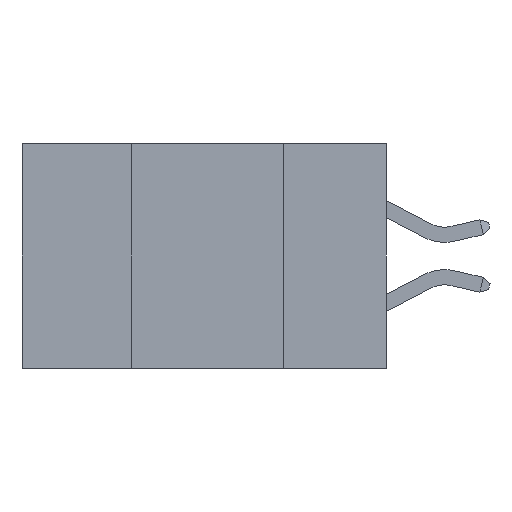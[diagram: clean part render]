
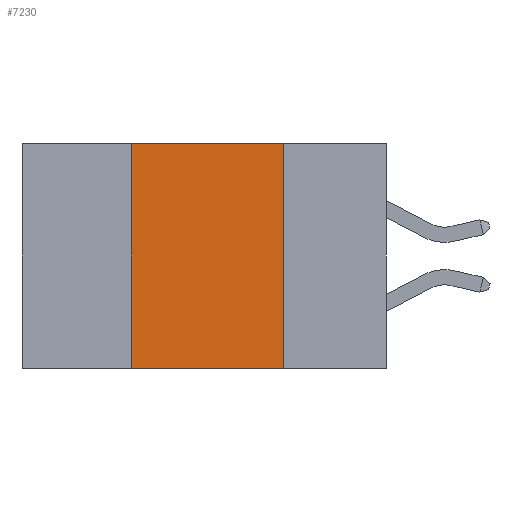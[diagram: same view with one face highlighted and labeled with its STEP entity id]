
A CAD part, left-side view. The second image highlights one B-rep face of the part: STEP entity #7230.
In plain terms, the highlighted planar face has unit normal (-1, 0, 0).
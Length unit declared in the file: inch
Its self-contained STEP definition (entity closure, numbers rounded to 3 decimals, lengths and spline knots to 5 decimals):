
#641 = EDGE_LOOP ( 'NONE', ( #16654, #2404, #4590, #13227 ) ) ;
#651 = EDGE_CURVE ( 'NONE', #1362, #14992, #16587, .T. ) ;
#781 = CARTESIAN_POINT ( 'NONE',  ( 0., 0.17, 0. ) ) ;
#1362 = VERTEX_POINT ( 'NONE', #781 ) ;
#2283 = DIRECTION ( 'NONE',  ( 0., -1., 0. ) ) ;
#2404 = ORIENTED_EDGE ( 'NONE', *, *, #9016, .F. ) ;
#4414 = DIRECTION ( 'NONE',  ( 0., 0., -1. ) ) ;
#4590 = ORIENTED_EDGE ( 'NONE', *, *, #5785, .F. ) ;
#5785 = EDGE_CURVE ( 'NONE', #12525, #13629, #13526, .T. ) ;
#5913 = CARTESIAN_POINT ( 'NONE',  ( 0., 0.42, -0.37 ) ) ;
#7230 = ADVANCED_FACE ( 'NONE', ( #9257 ), #9607, .F. ) ;
#7318 = VECTOR ( 'NONE', #2283, 39.37008 ) ;
#7525 = CARTESIAN_POINT ( 'NONE',  ( 0., 0.42, 0. ) ) ;
#7535 = CARTESIAN_POINT ( 'NONE',  ( 0., 0.42, -0.37 ) ) ;
#8121 = VECTOR ( 'NONE', #22055, 39.37008 ) ;
#9016 = EDGE_CURVE ( 'NONE', #13629, #1362, #20378, .T. ) ;
#9257 = FACE_OUTER_BOUND ( 'NONE', #641, .T. ) ;
#9265 = DIRECTION ( 'NONE',  ( 0., 0., 1. ) ) ;
#9607 = PLANE ( 'NONE',  #15747 ) ;
#10908 = CARTESIAN_POINT ( 'NONE',  ( 0., 0.6, 0. ) ) ;
#12525 = VERTEX_POINT ( 'NONE', #5913 ) ;
#13008 = CARTESIAN_POINT ( 'NONE',  ( 0., 0.6, 0. ) ) ;
#13227 = ORIENTED_EDGE ( 'NONE', *, *, #13850, .T. ) ;
#13471 = LINE ( 'NONE', #21646, #16906 ) ;
#13526 = LINE ( 'NONE', #7535, #14594 ) ;
#13629 = VERTEX_POINT ( 'NONE', #7525 ) ;
#13850 = EDGE_CURVE ( 'NONE', #12525, #14992, #13471, .T. ) ;
#14594 = VECTOR ( 'NONE', #9265, 39.37008 ) ;
#14720 = DIRECTION ( 'NONE',  ( 1., 0., 0. ) ) ;
#14992 = VERTEX_POINT ( 'NONE', #21101 ) ;
#15747 = AXIS2_PLACEMENT_3D ( 'NONE', #13008, #14720, #4414 ) ;
#16483 = DIRECTION ( 'NONE',  ( 0., -1., 0. ) ) ;
#16587 = LINE ( 'NONE', #17990, #8121 ) ;
#16654 = ORIENTED_EDGE ( 'NONE', *, *, #651, .F. ) ;
#16906 = VECTOR ( 'NONE', #16483, 39.37008 ) ;
#17990 = CARTESIAN_POINT ( 'NONE',  ( 0., 0.17, -0.37 ) ) ;
#20378 = LINE ( 'NONE', #10908, #7318 ) ;
#21101 = CARTESIAN_POINT ( 'NONE',  ( 0., 0.17, -0.37 ) ) ;
#21646 = CARTESIAN_POINT ( 'NONE',  ( 0., 0.6, -0.37 ) ) ;
#22055 = DIRECTION ( 'NONE',  ( 0., 0., -1. ) ) ;
